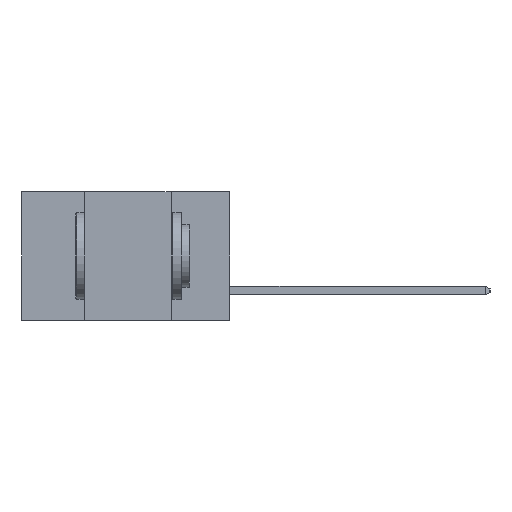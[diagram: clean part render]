
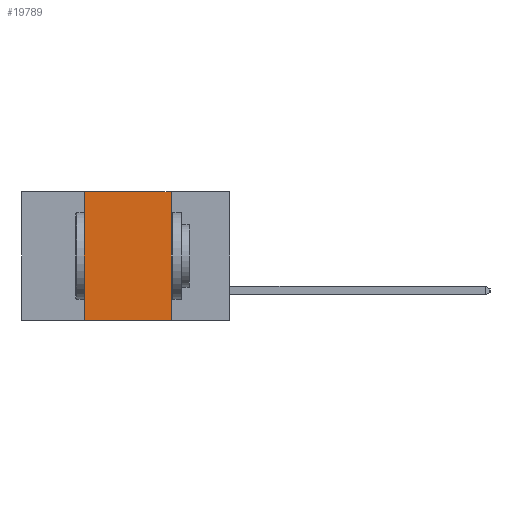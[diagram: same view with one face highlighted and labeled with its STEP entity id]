
A CAD part, left-side view. The second image highlights one B-rep face of the part: STEP entity #19789.
In plain terms, the highlighted planar face has unit normal (-1, 0, 0).
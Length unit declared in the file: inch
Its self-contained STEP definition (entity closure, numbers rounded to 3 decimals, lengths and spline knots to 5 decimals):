
#528 = ORIENTED_EDGE ( 'NONE', *, *, #10963, .F. ) ;
#656 = VECTOR ( 'NONE', #19416, 39.37008 ) ;
#1143 = CARTESIAN_POINT ( 'NONE',  ( 0., 0.17, 0. ) ) ;
#1201 = CARTESIAN_POINT ( 'NONE',  ( 0., 0.6, 0. ) ) ;
#2581 = VERTEX_POINT ( 'NONE', #9062 ) ;
#4020 = CARTESIAN_POINT ( 'NONE',  ( 0., 0.42, 0. ) ) ;
#6634 = FACE_OUTER_BOUND ( 'NONE', #27032, .T. ) ;
#7007 = ORIENTED_EDGE ( 'NONE', *, *, #9514, .T. ) ;
#7404 = AXIS2_PLACEMENT_3D ( 'NONE', #10521, #8437, #23785 ) ;
#7598 = DIRECTION ( 'NONE',  ( 0., -1., 0. ) ) ;
#8437 = DIRECTION ( 'NONE',  ( 1., 0., 0. ) ) ;
#9062 = CARTESIAN_POINT ( 'NONE',  ( 0., 0.17, 0. ) ) ;
#9514 = EDGE_CURVE ( 'NONE', #10756, #14876, #16218, .T. ) ;
#9586 = EDGE_CURVE ( 'NONE', #23867, #2581, #14802, .T. ) ;
#10521 = CARTESIAN_POINT ( 'NONE',  ( 0., 0.6, 0. ) ) ;
#10756 = VERTEX_POINT ( 'NONE', #14204 ) ;
#10963 = EDGE_CURVE ( 'NONE', #10756, #23867, #11548, .T. ) ;
#11548 = LINE ( 'NONE', #4020, #656 ) ;
#14204 = CARTESIAN_POINT ( 'NONE',  ( 0., 0.42, -0.37 ) ) ;
#14315 = DIRECTION ( 'NONE',  ( 0., 0., -1. ) ) ;
#14802 = LINE ( 'NONE', #1201, #19961 ) ;
#14876 = VERTEX_POINT ( 'NONE', #15978 ) ;
#15978 = CARTESIAN_POINT ( 'NONE',  ( 0., 0.17, -0.37 ) ) ;
#16029 = ORIENTED_EDGE ( 'NONE', *, *, #22781, .F. ) ;
#16218 = LINE ( 'NONE', #20812, #26948 ) ;
#19416 = DIRECTION ( 'NONE',  ( 0., 0., 1. ) ) ;
#19789 = ADVANCED_FACE ( 'NONE', ( #6634 ), #21624, .F. ) ;
#19961 = VECTOR ( 'NONE', #20999, 39.37008 ) ;
#20812 = CARTESIAN_POINT ( 'NONE',  ( 0., 0.6, -0.37 ) ) ;
#20999 = DIRECTION ( 'NONE',  ( 0., -1., 0. ) ) ;
#21624 = PLANE ( 'NONE',  #7404 ) ;
#21981 = VECTOR ( 'NONE', #14315, 39.37008 ) ;
#22636 = LINE ( 'NONE', #1143, #21981 ) ;
#22781 = EDGE_CURVE ( 'NONE', #2581, #14876, #22636, .T. ) ;
#23785 = DIRECTION ( 'NONE',  ( 0., 0., -1. ) ) ;
#23867 = VERTEX_POINT ( 'NONE', #26772 ) ;
#26772 = CARTESIAN_POINT ( 'NONE',  ( 0., 0.42, 0. ) ) ;
#26948 = VECTOR ( 'NONE', #7598, 39.37008 ) ;
#27032 = EDGE_LOOP ( 'NONE', ( #16029, #27407, #528, #7007 ) ) ;
#27407 = ORIENTED_EDGE ( 'NONE', *, *, #9586, .F. ) ;
